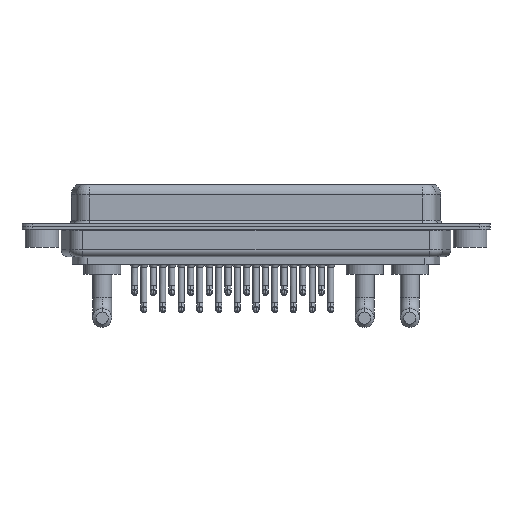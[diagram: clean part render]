
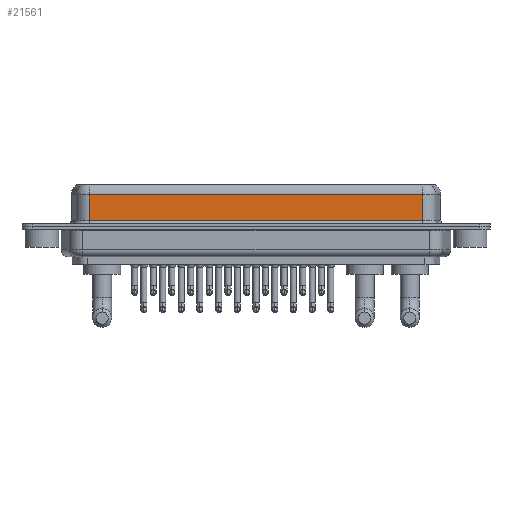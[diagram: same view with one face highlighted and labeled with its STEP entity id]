
A CAD part, front view. The second image highlights one B-rep face of the part: STEP entity #21561.
In plain terms, the highlighted planar face has unit normal (0, -1, 0).
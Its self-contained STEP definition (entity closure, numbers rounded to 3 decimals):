
#408 = CARTESIAN_POINT ( 'NONE',  ( 7.038, -3.95, 6.4 ) ) ;
#719 = EDGE_CURVE ( 'NONE', #3708, #17570, #5925, .T. ) ;
#831 = CARTESIAN_POINT ( 'NONE',  ( 7.038, -3.95, 0.9 ) ) ;
#3282 = EDGE_CURVE ( 'NONE', #17570, #14590, #22139, .T. ) ;
#3667 = PLANE ( 'NONE',  #10045 ) ;
#3708 = VERTEX_POINT ( 'NONE', #3989 ) ;
#3989 = CARTESIAN_POINT ( 'NONE',  ( 7.038, -3.95, 4.65 ) ) ;
#4016 = DIRECTION ( 'NONE',  ( 1., 0., 0. ) ) ;
#4580 = CARTESIAN_POINT ( 'NONE',  ( 56.462, -3.95, 6.4 ) ) ;
#5056 = DIRECTION ( 'NONE',  ( -1., 0., 0. ) ) ;
#5586 = CARTESIAN_POINT ( 'NONE',  ( 56.462, -3.95, 6.4 ) ) ;
#5925 = LINE ( 'NONE', #408, #22662 ) ;
#6034 = EDGE_CURVE ( 'NONE', #14715, #3708, #12533, .T. ) ;
#6441 = CARTESIAN_POINT ( 'NONE',  ( 56.462, -3.95, 4.65 ) ) ;
#8571 = EDGE_LOOP ( 'NONE', ( #18299, #17018, #20258, #21574 ) ) ;
#8581 = DIRECTION ( 'NONE',  ( 0., 0., -1. ) ) ;
#8934 = CARTESIAN_POINT ( 'NONE',  ( 56.462, -3.95, 4.65 ) ) ;
#8990 = FACE_OUTER_BOUND ( 'NONE', #8571, .T. ) ;
#10045 = AXIS2_PLACEMENT_3D ( 'NONE', #5586, #10563, #21689 ) ;
#10563 = DIRECTION ( 'NONE',  ( 0., 1., 0. ) ) ;
#10603 = EDGE_CURVE ( 'NONE', #14715, #14590, #16040, .T. ) ;
#11488 = VECTOR ( 'NONE', #8581, 1000. ) ;
#12533 = LINE ( 'NONE', #8934, #20641 ) ;
#14590 = VERTEX_POINT ( 'NONE', #20360 ) ;
#14715 = VERTEX_POINT ( 'NONE', #6441 ) ;
#15092 = DIRECTION ( 'NONE',  ( 0., 0., -1. ) ) ;
#16040 = LINE ( 'NONE', #4580, #11488 ) ;
#16703 = CARTESIAN_POINT ( 'NONE',  ( 56.462, -3.95, 0.9 ) ) ;
#17018 = ORIENTED_EDGE ( 'NONE', *, *, #6034, .T. ) ;
#17570 = VERTEX_POINT ( 'NONE', #831 ) ;
#18299 = ORIENTED_EDGE ( 'NONE', *, *, #10603, .F. ) ;
#20258 = ORIENTED_EDGE ( 'NONE', *, *, #719, .T. ) ;
#20360 = CARTESIAN_POINT ( 'NONE',  ( 56.462, -3.95, 0.9 ) ) ;
#20641 = VECTOR ( 'NONE', #5056, 1000. ) ;
#21561 = ADVANCED_FACE ( 'NONE', ( #8990 ), #3667, .F. ) ;
#21574 = ORIENTED_EDGE ( 'NONE', *, *, #3282, .T. ) ;
#21689 = DIRECTION ( 'NONE',  ( 0., 0., 1. ) ) ;
#22139 = LINE ( 'NONE', #16703, #22895 ) ;
#22662 = VECTOR ( 'NONE', #15092, 1000. ) ;
#22895 = VECTOR ( 'NONE', #4016, 1000. ) ;
